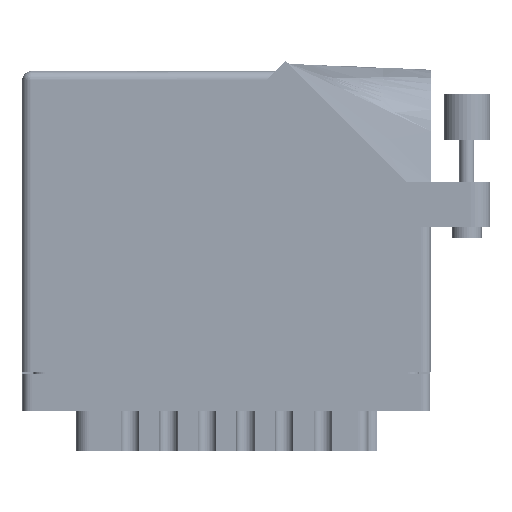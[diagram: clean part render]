
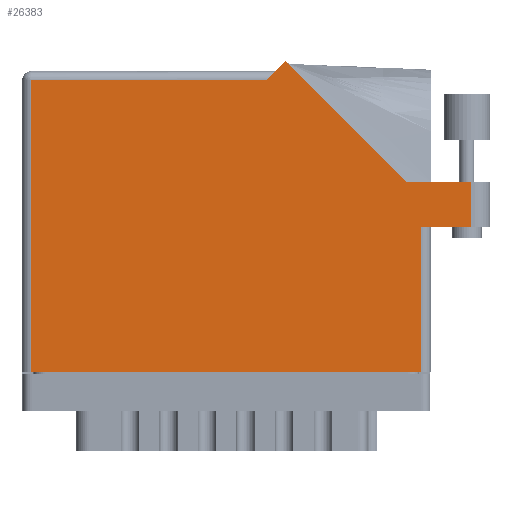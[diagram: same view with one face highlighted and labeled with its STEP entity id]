
A CAD part, front view. The second image highlights one B-rep face of the part: STEP entity #26383.
In plain terms, the highlighted face is planar.
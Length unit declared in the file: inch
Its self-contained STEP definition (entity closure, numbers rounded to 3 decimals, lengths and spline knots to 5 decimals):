
#3060 = VECTOR ( 'NONE', #88836, 39.37008 ) ;
#4402 = VECTOR ( 'NONE', #37394, 39.37008 ) ;
#4985 = CARTESIAN_POINT ( 'NONE',  ( 1.643, 1.968, 0. ) ) ;
#6646 = VERTEX_POINT ( 'NONE', #51792 ) ;
#6729 = DIRECTION ( 'NONE',  ( 0., -1., 0. ) ) ;
#6993 = ORIENTED_EDGE ( 'NONE', *, *, #90942, .T. ) ;
#7338 = VECTOR ( 'NONE', #22129, 39.37008 ) ;
#7363 = FACE_OUTER_BOUND ( 'NONE', #56745, .T. ) ;
#7403 = DIRECTION ( 'NONE',  ( 1., 0., 0. ) ) ;
#7513 = LINE ( 'NONE', #16489, #83859 ) ;
#7526 = ORIENTED_EDGE ( 'NONE', *, *, #77959, .T. ) ;
#8057 = VECTOR ( 'NONE', #6729, 39.37008 ) ;
#10342 = VECTOR ( 'NONE', #79390, 39.37008 ) ;
#11801 = VERTEX_POINT ( 'NONE', #87990 ) ;
#11981 = VERTEX_POINT ( 'NONE', #12360 ) ;
#12360 = CARTESIAN_POINT ( 'NONE',  ( 2.693, 0., 0. ) ) ;
#12627 = CARTESIAN_POINT ( 'NONE',  ( 3.03, 1.287, 0. ) ) ;
#13023 = VERTEX_POINT ( 'NONE', #21634 ) ;
#16489 = CARTESIAN_POINT ( 'NONE',  ( 2.693, 0.98, 0. ) ) ;
#17269 = PLANE ( 'NONE',  #75110 ) ;
#19128 = EDGE_CURVE ( 'NONE', #70698, #6646, #41337, .T. ) ;
#21634 = CARTESIAN_POINT ( 'NONE',  ( 0.062, 0., 0. ) ) ;
#22129 = DIRECTION ( 'NONE',  ( 0., 1., 0. ) ) ;
#22269 = EDGE_CURVE ( 'NONE', #88176, #13023, #46285, .T. ) ;
#22436 = CARTESIAN_POINT ( 'NONE',  ( 3.03, 1.287, 0. ) ) ;
#24441 = ORIENTED_EDGE ( 'NONE', *, *, #52356, .T. ) ;
#25440 = ORIENTED_EDGE ( 'NONE', *, *, #87736, .T. ) ;
#26383 = ADVANCED_FACE ( 'NONE', ( #7363 ), #17269, .F. ) ;
#28435 = VERTEX_POINT ( 'NONE', #36576 ) ;
#29058 = EDGE_CURVE ( 'NONE', #6646, #60570, #49588, .T. ) ;
#29178 = DIRECTION ( 'NONE',  ( -1., 0., 0. ) ) ;
#29212 = ORIENTED_EDGE ( 'NONE', *, *, #22269, .T. ) ;
#29513 = LINE ( 'NONE', #91379, #72125 ) ;
#31297 = DIRECTION ( 'NONE',  ( 0., 1., 0. ) ) ;
#32301 = LINE ( 'NONE', #72338, #63655 ) ;
#34980 = DIRECTION ( 'NONE',  ( 1., 0., 0. ) ) ;
#36576 = CARTESIAN_POINT ( 'NONE',  ( 3.03, 0.98, 0. ) ) ;
#36845 = ORIENTED_EDGE ( 'NONE', *, *, #29058, .T. ) ;
#37394 = DIRECTION ( 'NONE',  ( -1., 0., 0. ) ) ;
#38156 = LINE ( 'NONE', #72175, #4402 ) ;
#39514 = VECTOR ( 'NONE', #29178, 39.37008 ) ;
#40692 = VERTEX_POINT ( 'NONE', #12627 ) ;
#41337 = LINE ( 'NONE', #81666, #3060 ) ;
#42662 = EDGE_CURVE ( 'NONE', #11801, #28435, #29513, .T. ) ;
#46285 = LINE ( 'NONE', #83644, #8057 ) ;
#48149 = CARTESIAN_POINT ( 'NONE',  ( 0.062, 1.968, 0. ) ) ;
#49588 = LINE ( 'NONE', #65867, #10342 ) ;
#51792 = CARTESIAN_POINT ( 'NONE',  ( 1.77571, 2.10071, 0. ) ) ;
#52356 = EDGE_CURVE ( 'NONE', #11981, #11801, #7513, .T. ) ;
#56745 = EDGE_LOOP ( 'NONE', ( #70234, #81776, #7526, #82045, #36845, #6993, #29212, #25440, #24441 ) ) ;
#56787 = CARTESIAN_POINT ( 'NONE',  ( 0., 1.968, 0. ) ) ;
#59295 = DIRECTION ( 'NONE',  ( -1., 0., 0. ) ) ;
#60570 = VERTEX_POINT ( 'NONE', #4985 ) ;
#63655 = VECTOR ( 'NONE', #7403, 39.37008 ) ;
#65867 = CARTESIAN_POINT ( 'NONE',  ( 1.705, 2.03, 0. ) ) ;
#67443 = CARTESIAN_POINT ( 'NONE',  ( 0., 2.03, 0. ) ) ;
#70234 = ORIENTED_EDGE ( 'NONE', *, *, #42662, .T. ) ;
#70698 = VERTEX_POINT ( 'NONE', #81989 ) ;
#72125 = VECTOR ( 'NONE', #34980, 39.37008 ) ;
#72175 = CARTESIAN_POINT ( 'NONE',  ( 3.155, 1.287, 0. ) ) ;
#72338 = CARTESIAN_POINT ( 'NONE',  ( 0., 0., 0. ) ) ;
#75110 = AXIS2_PLACEMENT_3D ( 'NONE', #67443, #87502, #59295 ) ;
#77959 = EDGE_CURVE ( 'NONE', #40692, #70698, #38156, .T. ) ;
#79195 = LINE ( 'NONE', #22436, #7338 ) ;
#79390 = DIRECTION ( 'NONE',  ( -0.707, -0.707, 0. ) ) ;
#80069 = EDGE_CURVE ( 'NONE', #28435, #40692, #79195, .T. ) ;
#81666 = CARTESIAN_POINT ( 'NONE',  ( 2.58942, 1.287, 0. ) ) ;
#81776 = ORIENTED_EDGE ( 'NONE', *, *, #80069, .T. ) ;
#81989 = CARTESIAN_POINT ( 'NONE',  ( 2.58942, 1.287, 0. ) ) ;
#82045 = ORIENTED_EDGE ( 'NONE', *, *, #19128, .T. ) ;
#83644 = CARTESIAN_POINT ( 'NONE',  ( 0.062, 0., 0. ) ) ;
#83859 = VECTOR ( 'NONE', #31297, 39.37008 ) ;
#84353 = LINE ( 'NONE', #56787, #39514 ) ;
#87502 = DIRECTION ( 'NONE',  ( 0., 0., -1. ) ) ;
#87736 = EDGE_CURVE ( 'NONE', #13023, #11981, #32301, .T. ) ;
#87990 = CARTESIAN_POINT ( 'NONE',  ( 2.693, 0.98, 0. ) ) ;
#88176 = VERTEX_POINT ( 'NONE', #48149 ) ;
#88836 = DIRECTION ( 'NONE',  ( -0.707, 0.707, 0. ) ) ;
#90942 = EDGE_CURVE ( 'NONE', #60570, #88176, #84353, .T. ) ;
#91379 = CARTESIAN_POINT ( 'NONE',  ( 2.755, 0.98, 0. ) ) ;
